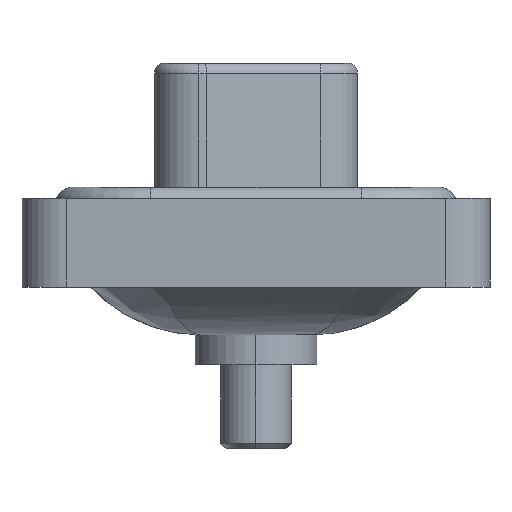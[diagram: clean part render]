
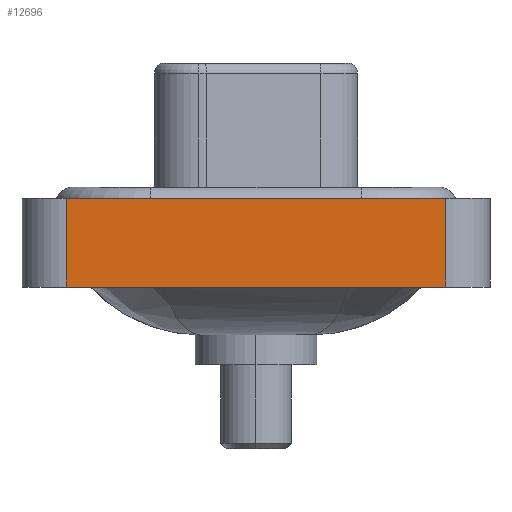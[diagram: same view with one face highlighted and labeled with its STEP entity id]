
A CAD part, left-side view. The second image highlights one B-rep face of the part: STEP entity #12696.
In plain terms, the highlighted planar face has unit normal (-1, 0, 0).
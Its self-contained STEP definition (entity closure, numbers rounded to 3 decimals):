
#24 = EDGE_CURVE ( 'NONE', #1570, #3371, #8582, .T. ) ;
#100 = ORIENTED_EDGE ( 'NONE', *, *, #1186, .F. ) ;
#1186 = EDGE_CURVE ( 'NONE', #1570, #14117, #2061, .T. ) ;
#1201 = CARTESIAN_POINT ( 'NONE',  ( -7.25, -8.55, -3.6 ) ) ;
#1570 = VERTEX_POINT ( 'NONE', #5434 ) ;
#1799 = LINE ( 'NONE', #5025, #11768 ) ;
#2025 = EDGE_LOOP ( 'NONE', ( #9895, #4529, #100, #13876 ) ) ;
#2061 = LINE ( 'NONE', #6695, #6891 ) ;
#3290 = PLANE ( 'NONE',  #11064 ) ;
#3353 = VECTOR ( 'NONE', #12182, 1000. ) ;
#3371 = VERTEX_POINT ( 'NONE', #11387 ) ;
#3564 = VERTEX_POINT ( 'NONE', #6964 ) ;
#3881 = CARTESIAN_POINT ( 'NONE',  ( -7.25, -8.55, 0.4 ) ) ;
#4001 = VECTOR ( 'NONE', #13531, 1000. ) ;
#4529 = ORIENTED_EDGE ( 'NONE', *, *, #8571, .F. ) ;
#5025 = CARTESIAN_POINT ( 'NONE',  ( -7.25, -8.55, -3.6 ) ) ;
#5103 = DIRECTION ( 'NONE',  ( 0., 0., 1. ) ) ;
#5434 = CARTESIAN_POINT ( 'NONE',  ( -7.25, 8.55, -3.6 ) ) ;
#6695 = CARTESIAN_POINT ( 'NONE',  ( -7.25, 8.55, -3.6 ) ) ;
#6891 = VECTOR ( 'NONE', #11419, 1000. ) ;
#6964 = CARTESIAN_POINT ( 'NONE',  ( -7.25, -8.55, 0.4 ) ) ;
#8571 = EDGE_CURVE ( 'NONE', #14117, #3564, #8848, .T. ) ;
#8582 = LINE ( 'NONE', #13309, #4001 ) ;
#8848 = LINE ( 'NONE', #3881, #3353 ) ;
#9001 = EDGE_CURVE ( 'NONE', #3371, #3564, #1799, .T. ) ;
#9240 = DIRECTION ( 'NONE',  ( -1., 0., 0. ) ) ;
#9895 = ORIENTED_EDGE ( 'NONE', *, *, #9001, .T. ) ;
#10405 = DIRECTION ( 'NONE',  ( 0., 0., 1. ) ) ;
#11064 = AXIS2_PLACEMENT_3D ( 'NONE', #1201, #9240, #10405 ) ;
#11387 = CARTESIAN_POINT ( 'NONE',  ( -7.25, -8.55, -3.6 ) ) ;
#11419 = DIRECTION ( 'NONE',  ( 0., 0., 1. ) ) ;
#11707 = CARTESIAN_POINT ( 'NONE',  ( -7.25, 8.55, 0.4 ) ) ;
#11768 = VECTOR ( 'NONE', #5103, 1000. ) ;
#12182 = DIRECTION ( 'NONE',  ( 0., -1., 0. ) ) ;
#12696 = ADVANCED_FACE ( 'NONE', ( #12814 ), #3290, .T. ) ;
#12814 = FACE_OUTER_BOUND ( 'NONE', #2025, .T. ) ;
#13309 = CARTESIAN_POINT ( 'NONE',  ( -7.25, -8.55, -3.6 ) ) ;
#13531 = DIRECTION ( 'NONE',  ( 0., -1., 0. ) ) ;
#13876 = ORIENTED_EDGE ( 'NONE', *, *, #24, .T. ) ;
#14117 = VERTEX_POINT ( 'NONE', #11707 ) ;
